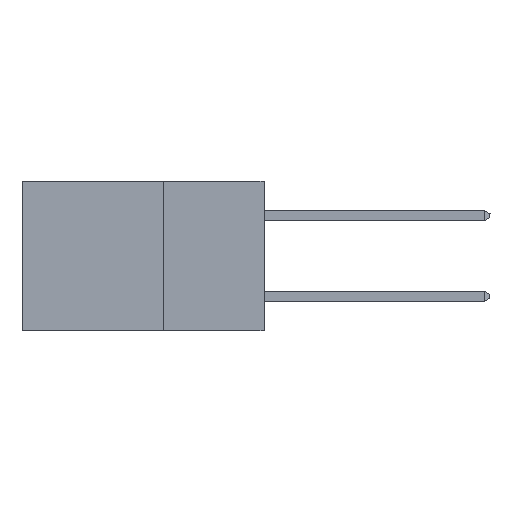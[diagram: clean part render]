
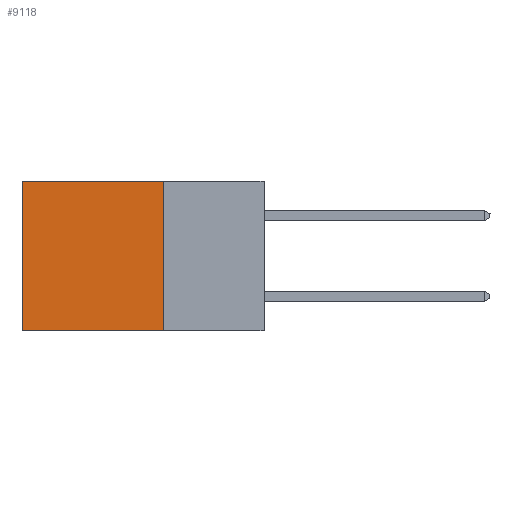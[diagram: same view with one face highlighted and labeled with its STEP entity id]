
A CAD part, left-side view. The second image highlights one B-rep face of the part: STEP entity #9118.
In plain terms, the highlighted planar face has unit normal (-1, 0, 0).
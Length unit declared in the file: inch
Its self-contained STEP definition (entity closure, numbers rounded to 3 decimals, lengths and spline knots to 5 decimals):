
#2246 = ORIENTED_EDGE ( 'NONE', *, *, #11822, .F. ) ;
#2301 = EDGE_CURVE ( 'NONE', #11408, #15829, #22257, .T. ) ;
#2407 = LINE ( 'NONE', #17999, #4596 ) ;
#2570 = DIRECTION ( 'NONE',  ( 0., 0., -1. ) ) ;
#4332 = VECTOR ( 'NONE', #18948, 39.37008 ) ;
#4596 = VECTOR ( 'NONE', #7181, 39.37008 ) ;
#5318 = CARTESIAN_POINT ( 'NONE',  ( 0.298, 0.25, 0. ) ) ;
#6373 = CARTESIAN_POINT ( 'NONE',  ( 0.298, 0.6, 0. ) ) ;
#6724 = LINE ( 'NONE', #5318, #22480 ) ;
#6886 = CARTESIAN_POINT ( 'NONE',  ( 0.298, 0.25, 0. ) ) ;
#7181 = DIRECTION ( 'NONE',  ( 0., 1., 0. ) ) ;
#7427 = EDGE_LOOP ( 'NONE', ( #21921, #2246, #21450, #8106 ) ) ;
#7721 = CARTESIAN_POINT ( 'NONE',  ( 0.298, 0.25, 0. ) ) ;
#7728 = CARTESIAN_POINT ( 'NONE',  ( 0.298, 0.6, 0. ) ) ;
#7907 = LINE ( 'NONE', #6886, #4332 ) ;
#8106 = ORIENTED_EDGE ( 'NONE', *, *, #12660, .T. ) ;
#8892 = DIRECTION ( 'NONE',  ( 0., 0., -1. ) ) ;
#9118 = ADVANCED_FACE ( 'NONE', ( #20981 ), #19182, .F. ) ;
#10382 = DIRECTION ( 'NONE',  ( 0., 0., -1. ) ) ;
#10625 = CARTESIAN_POINT ( 'NONE',  ( 0.298, 0.25, 0. ) ) ;
#11115 = CARTESIAN_POINT ( 'NONE',  ( 0.298, 0.25, -0.37 ) ) ;
#11240 = VECTOR ( 'NONE', #2570, 39.37008 ) ;
#11408 = VERTEX_POINT ( 'NONE', #6373 ) ;
#11822 = EDGE_CURVE ( 'NONE', #20536, #15829, #2407, .T. ) ;
#12353 = DIRECTION ( 'NONE',  ( 1., 0., 0. ) ) ;
#12362 = AXIS2_PLACEMENT_3D ( 'NONE', #10625, #12353, #10382 ) ;
#12660 = EDGE_CURVE ( 'NONE', #14311, #11408, #7907, .T. ) ;
#14045 = CARTESIAN_POINT ( 'NONE',  ( 0.298, 0.6, -0.37 ) ) ;
#14311 = VERTEX_POINT ( 'NONE', #7721 ) ;
#15829 = VERTEX_POINT ( 'NONE', #14045 ) ;
#17536 = EDGE_CURVE ( 'NONE', #14311, #20536, #6724, .T. ) ;
#17999 = CARTESIAN_POINT ( 'NONE',  ( 0.298, 0.25, -0.37 ) ) ;
#18948 = DIRECTION ( 'NONE',  ( 0., 1., 0. ) ) ;
#19182 = PLANE ( 'NONE',  #12362 ) ;
#20536 = VERTEX_POINT ( 'NONE', #11115 ) ;
#20981 = FACE_OUTER_BOUND ( 'NONE', #7427, .T. ) ;
#21450 = ORIENTED_EDGE ( 'NONE', *, *, #17536, .F. ) ;
#21921 = ORIENTED_EDGE ( 'NONE', *, *, #2301, .T. ) ;
#22257 = LINE ( 'NONE', #7728, #11240 ) ;
#22480 = VECTOR ( 'NONE', #8892, 39.37008 ) ;
